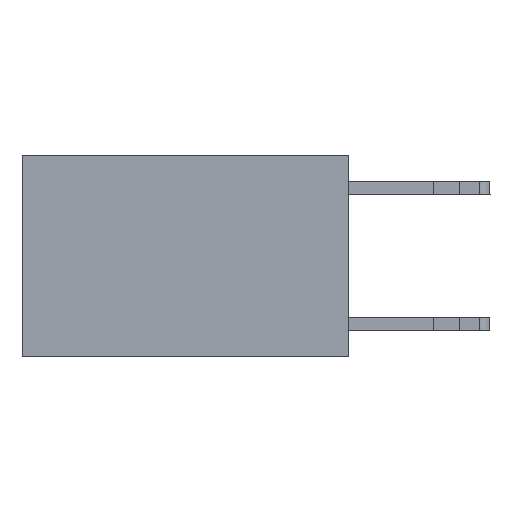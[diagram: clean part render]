
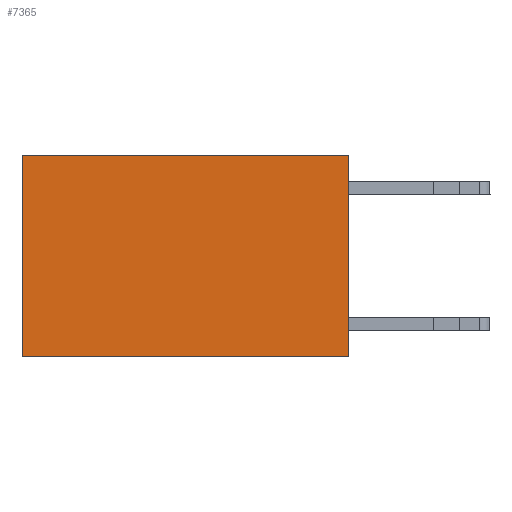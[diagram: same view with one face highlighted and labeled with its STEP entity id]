
A CAD part, left-side view. The second image highlights one B-rep face of the part: STEP entity #7365.
In plain terms, the highlighted planar face has unit normal (-1, 0, 0).
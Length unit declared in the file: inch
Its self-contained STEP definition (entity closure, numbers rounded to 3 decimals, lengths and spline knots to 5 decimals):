
#517 = VERTEX_POINT ( 'NONE', #23555 ) ;
#1447 = CARTESIAN_POINT ( 'NONE',  ( 0.2625, 0., -0.37 ) ) ;
#1568 = ORIENTED_EDGE ( 'NONE', *, *, #8658, .T. ) ;
#3200 = VECTOR ( 'NONE', #3563, 39.37008 ) ;
#3563 = DIRECTION ( 'NONE',  ( 0., 0., -1. ) ) ;
#4312 = AXIS2_PLACEMENT_3D ( 'NONE', #5643, #20776, #7814 ) ;
#5643 = CARTESIAN_POINT ( 'NONE',  ( 0.2625, 0., 0. ) ) ;
#6347 = ORIENTED_EDGE ( 'NONE', *, *, #27321, .T. ) ;
#7365 = ADVANCED_FACE ( 'NONE', ( #22782 ), #16433, .F. ) ;
#7486 = VECTOR ( 'NONE', #19900, 39.37008 ) ;
#7767 = EDGE_CURVE ( 'NONE', #23219, #11940, #24817, .T. ) ;
#7814 = DIRECTION ( 'NONE',  ( 0., 0., -1. ) ) ;
#8658 = EDGE_CURVE ( 'NONE', #517, #11940, #20994, .T. ) ;
#11940 = VERTEX_POINT ( 'NONE', #14830 ) ;
#14037 = LINE ( 'NONE', #27385, #3200 ) ;
#14390 = CARTESIAN_POINT ( 'NONE',  ( 0.2625, 0.6, 0. ) ) ;
#14830 = CARTESIAN_POINT ( 'NONE',  ( 0.2625, 0.6, -0.37 ) ) ;
#16283 = CARTESIAN_POINT ( 'NONE',  ( 0.2625, 0., 0. ) ) ;
#16433 = PLANE ( 'NONE',  #4312 ) ;
#16732 = EDGE_LOOP ( 'NONE', ( #1568, #25672, #27171, #6347 ) ) ;
#17153 = CARTESIAN_POINT ( 'NONE',  ( 0.2625, 0., 0. ) ) ;
#17730 = CARTESIAN_POINT ( 'NONE',  ( 0.2625, 0., -0.37 ) ) ;
#19900 = DIRECTION ( 'NONE',  ( 0., 1., 0. ) ) ;
#20231 = EDGE_CURVE ( 'NONE', #26231, #23219, #14037, .T. ) ;
#20314 = VECTOR ( 'NONE', #27428, 39.37008 ) ;
#20776 = DIRECTION ( 'NONE',  ( 1., 0., 0. ) ) ;
#20994 = LINE ( 'NONE', #14390, #20314 ) ;
#22746 = DIRECTION ( 'NONE',  ( 0., 1., 0. ) ) ;
#22782 = FACE_OUTER_BOUND ( 'NONE', #16732, .T. ) ;
#23138 = VECTOR ( 'NONE', #22746, 39.37008 ) ;
#23219 = VERTEX_POINT ( 'NONE', #1447 ) ;
#23555 = CARTESIAN_POINT ( 'NONE',  ( 0.2625, 0.6, 0. ) ) ;
#23854 = LINE ( 'NONE', #16283, #23138 ) ;
#24817 = LINE ( 'NONE', #17730, #7486 ) ;
#25672 = ORIENTED_EDGE ( 'NONE', *, *, #7767, .F. ) ;
#26231 = VERTEX_POINT ( 'NONE', #17153 ) ;
#27171 = ORIENTED_EDGE ( 'NONE', *, *, #20231, .F. ) ;
#27321 = EDGE_CURVE ( 'NONE', #26231, #517, #23854, .T. ) ;
#27385 = CARTESIAN_POINT ( 'NONE',  ( 0.2625, 0., 0. ) ) ;
#27428 = DIRECTION ( 'NONE',  ( 0., 0., -1. ) ) ;
